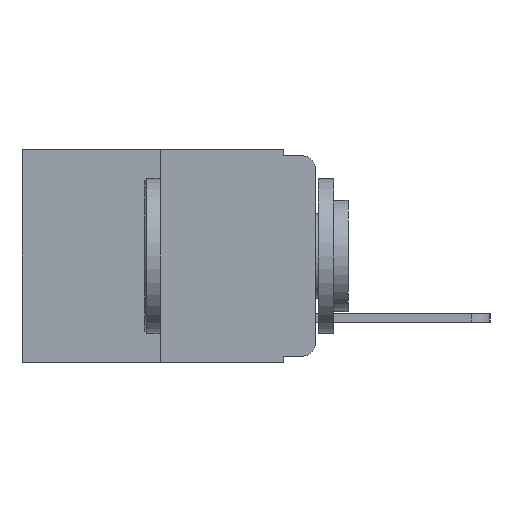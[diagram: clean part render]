
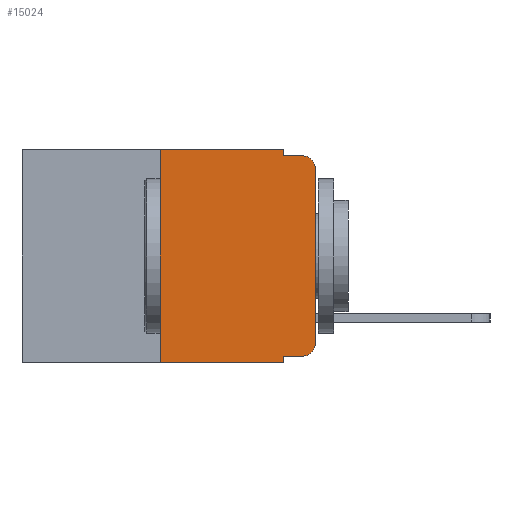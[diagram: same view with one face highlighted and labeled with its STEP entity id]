
A CAD part, left-side view. The second image highlights one B-rep face of the part: STEP entity #15024.
In plain terms, the highlighted planar face has unit normal (-1, 0, 0).
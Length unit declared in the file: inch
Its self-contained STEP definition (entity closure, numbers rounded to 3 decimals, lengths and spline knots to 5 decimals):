
#163 = CIRCLE ( 'NONE', #3143, 0.02 ) ;
#210 = LINE ( 'NONE', #4143, #16900 ) ;
#796 = CARTESIAN_POINT ( 'NONE',  ( 0., 0.051, 0. ) ) ;
#1052 = CARTESIAN_POINT ( 'NONE',  ( 0., 0.051, -0.333 ) ) ;
#1126 = CARTESIAN_POINT ( 'NONE',  ( 0., 0.051, -0.333 ) ) ;
#1305 = DIRECTION ( 'NONE',  ( 0., 0., 1. ) ) ;
#1587 = EDGE_CURVE ( 'NONE', #4537, #4564, #210, .T. ) ;
#1652 = VECTOR ( 'NONE', #12805, 39.37008 ) ;
#1906 = ORIENTED_EDGE ( 'NONE', *, *, #1587, .T. ) ;
#2054 = DIRECTION ( 'NONE',  ( 0., 0., -1. ) ) ;
#2063 = CARTESIAN_POINT ( 'NONE',  ( 0., 0.051, -0.01 ) ) ;
#2232 = CIRCLE ( 'NONE', #10250, 0.02 ) ;
#2377 = DIRECTION ( 'NONE',  ( 0., 0., -1. ) ) ;
#2495 = VECTOR ( 'NONE', #6412, 39.37008 ) ;
#2632 = VECTOR ( 'NONE', #6221, 39.37008 ) ;
#2662 = CARTESIAN_POINT ( 'NONE',  ( 0., 0.25, 0. ) ) ;
#2846 = DIRECTION ( 'NONE',  ( -1., 0., 0. ) ) ;
#2884 = VERTEX_POINT ( 'NONE', #12791 ) ;
#2976 = VERTEX_POINT ( 'NONE', #2063 ) ;
#3143 = AXIS2_PLACEMENT_3D ( 'NONE', #10843, #2846, #12118 ) ;
#3448 = CARTESIAN_POINT ( 'NONE',  ( 0., 0.051, 0. ) ) ;
#3948 = DIRECTION ( 'NONE',  ( 0., 0., 1. ) ) ;
#4033 = CARTESIAN_POINT ( 'NONE',  ( 0., 0., -0.03 ) ) ;
#4056 = ORIENTED_EDGE ( 'NONE', *, *, #6465, .T. ) ;
#4143 = CARTESIAN_POINT ( 'NONE',  ( 0., 0., 0. ) ) ;
#4537 = VERTEX_POINT ( 'NONE', #5077 ) ;
#4564 = VERTEX_POINT ( 'NONE', #4033 ) ;
#5066 = CARTESIAN_POINT ( 'NONE',  ( 0., 0.051, -0.01 ) ) ;
#5077 = CARTESIAN_POINT ( 'NONE',  ( 0., 0., -0.313 ) ) ;
#5438 = CARTESIAN_POINT ( 'NONE',  ( 0., 0.051, 0. ) ) ;
#5509 = ORIENTED_EDGE ( 'NONE', *, *, #16039, .T. ) ;
#5639 = VECTOR ( 'NONE', #2054, 39.37008 ) ;
#5854 = EDGE_LOOP ( 'NONE', ( #1906, #5509, #15922, #12872, #6376, #9898, #13272, #6789, #13695, #4056 ) ) ;
#6066 = LINE ( 'NONE', #3448, #5639 ) ;
#6221 = DIRECTION ( 'NONE',  ( 0., 0., -1. ) ) ;
#6376 = ORIENTED_EDGE ( 'NONE', *, *, #14436, .F. ) ;
#6412 = DIRECTION ( 'NONE',  ( 0., -1., 0. ) ) ;
#6465 = EDGE_CURVE ( 'NONE', #10093, #4537, #163, .T. ) ;
#6675 = LINE ( 'NONE', #796, #2632 ) ;
#6789 = ORIENTED_EDGE ( 'NONE', *, *, #10013, .F. ) ;
#6989 = VECTOR ( 'NONE', #16979, 39.37008 ) ;
#7573 = VERTEX_POINT ( 'NONE', #9079 ) ;
#7632 = DIRECTION ( 'NONE',  ( -1., 0., 0. ) ) ;
#7671 = CARTESIAN_POINT ( 'NONE',  ( 0., 0.02, -0.333 ) ) ;
#7716 = VERTEX_POINT ( 'NONE', #14625 ) ;
#8199 = VERTEX_POINT ( 'NONE', #1052 ) ;
#8220 = EDGE_CURVE ( 'NONE', #8199, #10093, #16508, .T. ) ;
#8390 = FACE_OUTER_BOUND ( 'NONE', #5854, .T. ) ;
#8797 = LINE ( 'NONE', #5066, #2495 ) ;
#9079 = CARTESIAN_POINT ( 'NONE',  ( 0., 0.02, -0.01 ) ) ;
#9090 = CARTESIAN_POINT ( 'NONE',  ( 0., 0.473, 0. ) ) ;
#9481 = VERTEX_POINT ( 'NONE', #5438 ) ;
#9680 = VECTOR ( 'NONE', #15592, 39.37008 ) ;
#9817 = VECTOR ( 'NONE', #1305, 39.37008 ) ;
#9898 = ORIENTED_EDGE ( 'NONE', *, *, #10881, .F. ) ;
#10013 = EDGE_CURVE ( 'NONE', #8199, #2884, #6066, .T. ) ;
#10093 = VERTEX_POINT ( 'NONE', #7671 ) ;
#10250 = AXIS2_PLACEMENT_3D ( 'NONE', #15411, #7632, #16677 ) ;
#10407 = DIRECTION ( 'NONE',  ( 1., 0., 0. ) ) ;
#10472 = LINE ( 'NONE', #10540, #6989 ) ;
#10540 = CARTESIAN_POINT ( 'NONE',  ( 0., 0.473, 0. ) ) ;
#10613 = LINE ( 'NONE', #10634, #9817 ) ;
#10634 = CARTESIAN_POINT ( 'NONE',  ( 0., 0.25, 0. ) ) ;
#10843 = CARTESIAN_POINT ( 'NONE',  ( 0., 0.02, -0.313 ) ) ;
#10881 = EDGE_CURVE ( 'NONE', #7716, #12635, #10613, .T. ) ;
#11738 = EDGE_CURVE ( 'NONE', #9481, #2976, #6675, .T. ) ;
#12118 = DIRECTION ( 'NONE',  ( 0., 0., -1. ) ) ;
#12249 = LINE ( 'NONE', #15379, #1652 ) ;
#12635 = VERTEX_POINT ( 'NONE', #2662 ) ;
#12791 = CARTESIAN_POINT ( 'NONE',  ( 0., 0.051, -0.343 ) ) ;
#12805 = DIRECTION ( 'NONE',  ( 0., -1., 0. ) ) ;
#12872 = ORIENTED_EDGE ( 'NONE', *, *, #11738, .F. ) ;
#12915 = PLANE ( 'NONE',  #15842 ) ;
#13272 = ORIENTED_EDGE ( 'NONE', *, *, #15409, .T. ) ;
#13695 = ORIENTED_EDGE ( 'NONE', *, *, #8220, .T. ) ;
#14325 = EDGE_CURVE ( 'NONE', #2976, #7573, #8797, .T. ) ;
#14436 = EDGE_CURVE ( 'NONE', #12635, #9481, #10472, .T. ) ;
#14625 = CARTESIAN_POINT ( 'NONE',  ( 0., 0.25, -0.343 ) ) ;
#15024 = ADVANCED_FACE ( 'NONE', ( #8390 ), #12915, .F. ) ;
#15379 = CARTESIAN_POINT ( 'NONE',  ( 0., 0.473, -0.343 ) ) ;
#15409 = EDGE_CURVE ( 'NONE', #7716, #2884, #12249, .T. ) ;
#15411 = CARTESIAN_POINT ( 'NONE',  ( 0., 0.02, -0.03 ) ) ;
#15592 = DIRECTION ( 'NONE',  ( 0., -1., 0. ) ) ;
#15842 = AXIS2_PLACEMENT_3D ( 'NONE', #9090, #10407, #2377 ) ;
#15922 = ORIENTED_EDGE ( 'NONE', *, *, #14325, .F. ) ;
#16039 = EDGE_CURVE ( 'NONE', #4564, #7573, #2232, .T. ) ;
#16508 = LINE ( 'NONE', #1126, #9680 ) ;
#16677 = DIRECTION ( 'NONE',  ( 0., 0., -1. ) ) ;
#16900 = VECTOR ( 'NONE', #3948, 39.37008 ) ;
#16979 = DIRECTION ( 'NONE',  ( 0., -1., 0. ) ) ;
